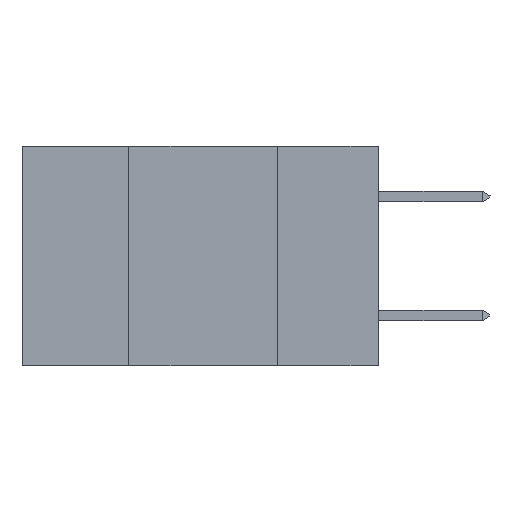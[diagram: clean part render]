
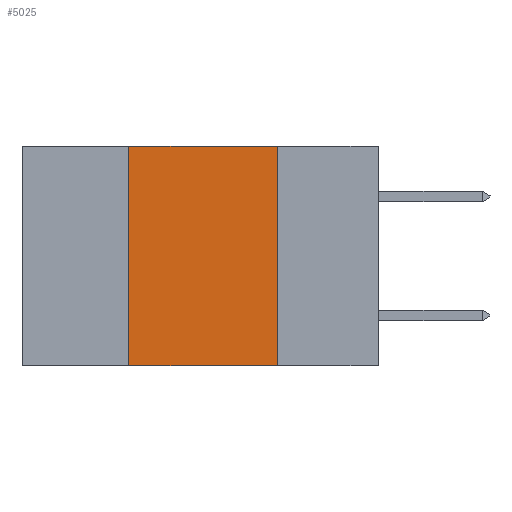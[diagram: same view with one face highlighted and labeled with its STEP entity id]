
A CAD part, left-side view. The second image highlights one B-rep face of the part: STEP entity #5025.
In plain terms, the highlighted planar face has unit normal (-1, 0, 0).
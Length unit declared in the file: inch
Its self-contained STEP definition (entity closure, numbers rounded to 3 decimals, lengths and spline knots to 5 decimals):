
#12 = LINE ( 'NONE', #6757, #4981 ) ;
#256 = CARTESIAN_POINT ( 'NONE',  ( 0., 0.6, 0. ) ) ;
#418 = EDGE_CURVE ( 'NONE', #8054, #7431, #12, .T. ) ;
#470 = ORIENTED_EDGE ( 'NONE', *, *, #418, .F. ) ;
#890 = EDGE_CURVE ( 'NONE', #5583, #8054, #9175, .T. ) ;
#1212 = VERTEX_POINT ( 'NONE', #1533 ) ;
#1379 = LINE ( 'NONE', #4354, #4733 ) ;
#1533 = CARTESIAN_POINT ( 'NONE',  ( 0., 0.17, -0.37 ) ) ;
#2340 = CARTESIAN_POINT ( 'NONE',  ( 0., 0.42, -0.37 ) ) ;
#2391 = DIRECTION ( 'NONE',  ( 0., 0., 1. ) ) ;
#2550 = DIRECTION ( 'NONE',  ( 1., 0., 0. ) ) ;
#2911 = EDGE_CURVE ( 'NONE', #5583, #1212, #5177, .T. ) ;
#2985 = EDGE_CURVE ( 'NONE', #7431, #1212, #1379, .T. ) ;
#2991 = PLANE ( 'NONE',  #4494 ) ;
#3542 = DIRECTION ( 'NONE',  ( 0., -1., 0. ) ) ;
#3999 = EDGE_LOOP ( 'NONE', ( #8978, #470, #7406, #5606 ) ) ;
#4354 = CARTESIAN_POINT ( 'NONE',  ( 0., 0.17, -0.37 ) ) ;
#4494 = AXIS2_PLACEMENT_3D ( 'NONE', #256, #2550, #7107 ) ;
#4733 = VECTOR ( 'NONE', #9765, 39.37008 ) ;
#4981 = VECTOR ( 'NONE', #6118, 39.37008 ) ;
#4989 = CARTESIAN_POINT ( 'NONE',  ( 0., 0.17, 0. ) ) ;
#5025 = ADVANCED_FACE ( 'NONE', ( #9799 ), #2991, .F. ) ;
#5177 = LINE ( 'NONE', #6615, #5656 ) ;
#5583 = VERTEX_POINT ( 'NONE', #7748 ) ;
#5606 = ORIENTED_EDGE ( 'NONE', *, *, #2911, .T. ) ;
#5656 = VECTOR ( 'NONE', #3542, 39.37008 ) ;
#6068 = CARTESIAN_POINT ( 'NONE',  ( 0., 0.42, 0. ) ) ;
#6118 = DIRECTION ( 'NONE',  ( 0., -1., 0. ) ) ;
#6123 = VECTOR ( 'NONE', #2391, 39.37008 ) ;
#6615 = CARTESIAN_POINT ( 'NONE',  ( 0., 0.6, -0.37 ) ) ;
#6757 = CARTESIAN_POINT ( 'NONE',  ( 0., 0.6, 0. ) ) ;
#7107 = DIRECTION ( 'NONE',  ( 0., 0., -1. ) ) ;
#7406 = ORIENTED_EDGE ( 'NONE', *, *, #890, .F. ) ;
#7431 = VERTEX_POINT ( 'NONE', #4989 ) ;
#7748 = CARTESIAN_POINT ( 'NONE',  ( 0., 0.42, -0.37 ) ) ;
#8054 = VERTEX_POINT ( 'NONE', #6068 ) ;
#8978 = ORIENTED_EDGE ( 'NONE', *, *, #2985, .F. ) ;
#9175 = LINE ( 'NONE', #2340, #6123 ) ;
#9765 = DIRECTION ( 'NONE',  ( 0., 0., -1. ) ) ;
#9799 = FACE_OUTER_BOUND ( 'NONE', #3999, .T. ) ;
